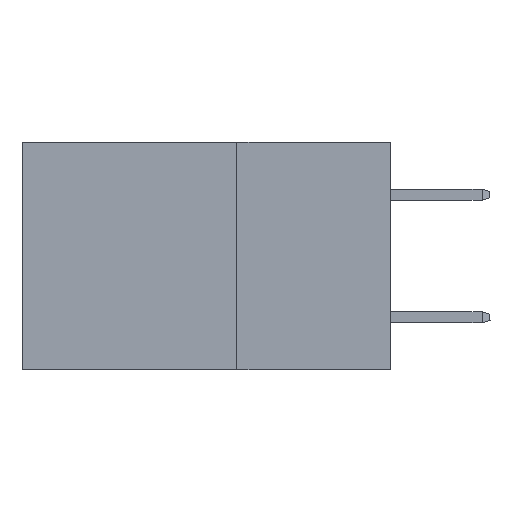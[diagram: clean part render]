
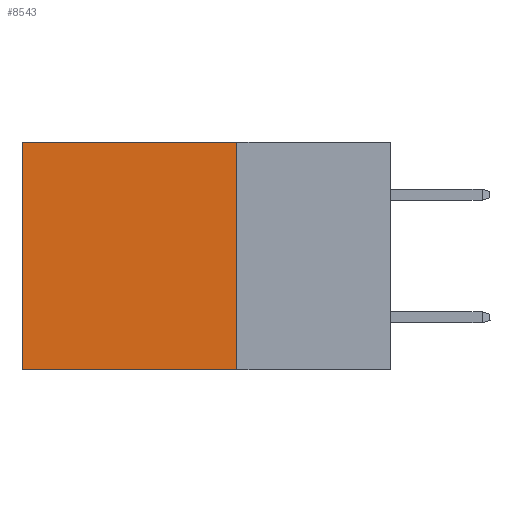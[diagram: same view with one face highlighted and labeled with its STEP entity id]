
A CAD part, left-side view. The second image highlights one B-rep face of the part: STEP entity #8543.
In plain terms, the highlighted planar face has unit normal (-1, 0, 0).
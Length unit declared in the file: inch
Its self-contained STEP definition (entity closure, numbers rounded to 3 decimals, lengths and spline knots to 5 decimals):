
#406 = ORIENTED_EDGE ( 'NONE', *, *, #8630, .T. ) ;
#531 = DIRECTION ( 'NONE',  ( 0., 1., 0. ) ) ;
#1273 = VERTEX_POINT ( 'NONE', #11655 ) ;
#3247 = PLANE ( 'NONE',  #36485 ) ;
#4452 = CARTESIAN_POINT ( 'NONE',  ( 0.2875, 0.6, 0. ) ) ;
#4723 = VERTEX_POINT ( 'NONE', #18147 ) ;
#8543 = ADVANCED_FACE ( 'NONE', ( #20619 ), #3247, .F. ) ;
#8567 = LINE ( 'NONE', #28787, #26486 ) ;
#8630 = EDGE_CURVE ( 'NONE', #20414, #22512, #21177, .T. ) ;
#10350 = LINE ( 'NONE', #19805, #29086 ) ;
#11655 = CARTESIAN_POINT ( 'NONE',  ( 0.2875, 0.6, -0.37 ) ) ;
#15192 = CARTESIAN_POINT ( 'NONE',  ( 0.2875, 0.25, 0. ) ) ;
#17057 = CARTESIAN_POINT ( 'NONE',  ( 0.2875, 0.25, 0. ) ) ;
#17347 = DIRECTION ( 'NONE',  ( 0., 0., -1. ) ) ;
#17901 = DIRECTION ( 'NONE',  ( 1., 0., 0. ) ) ;
#18147 = CARTESIAN_POINT ( 'NONE',  ( 0.2875, 0.25, -0.37 ) ) ;
#18988 = CARTESIAN_POINT ( 'NONE',  ( 0.2875, 0.25, -0.37 ) ) ;
#19805 = CARTESIAN_POINT ( 'NONE',  ( 0.2875, 0.25, 0. ) ) ;
#20414 = VERTEX_POINT ( 'NONE', #17057 ) ;
#20429 = EDGE_CURVE ( 'NONE', #22512, #1273, #8567, .T. ) ;
#20619 = FACE_OUTER_BOUND ( 'NONE', #26545, .T. ) ;
#21177 = LINE ( 'NONE', #30766, #26106 ) ;
#21640 = EDGE_CURVE ( 'NONE', #4723, #1273, #24771, .T. ) ;
#22280 = DIRECTION ( 'NONE',  ( 0., 1., 0. ) ) ;
#22512 = VERTEX_POINT ( 'NONE', #4452 ) ;
#24771 = LINE ( 'NONE', #18988, #29723 ) ;
#26106 = VECTOR ( 'NONE', #531, 39.37008 ) ;
#26289 = DIRECTION ( 'NONE',  ( 0., 0., -1. ) ) ;
#26486 = VECTOR ( 'NONE', #26289, 39.37008 ) ;
#26545 = EDGE_LOOP ( 'NONE', ( #33678, #33918, #36923, #406 ) ) ;
#28265 = DIRECTION ( 'NONE',  ( 0., 0., -1. ) ) ;
#28787 = CARTESIAN_POINT ( 'NONE',  ( 0.2875, 0.6, 0. ) ) ;
#29086 = VECTOR ( 'NONE', #28265, 39.37008 ) ;
#29723 = VECTOR ( 'NONE', #22280, 39.37008 ) ;
#30038 = EDGE_CURVE ( 'NONE', #20414, #4723, #10350, .T. ) ;
#30766 = CARTESIAN_POINT ( 'NONE',  ( 0.2875, 0.25, 0. ) ) ;
#33678 = ORIENTED_EDGE ( 'NONE', *, *, #20429, .T. ) ;
#33918 = ORIENTED_EDGE ( 'NONE', *, *, #21640, .F. ) ;
#36485 = AXIS2_PLACEMENT_3D ( 'NONE', #15192, #17901, #17347 ) ;
#36923 = ORIENTED_EDGE ( 'NONE', *, *, #30038, .F. ) ;
